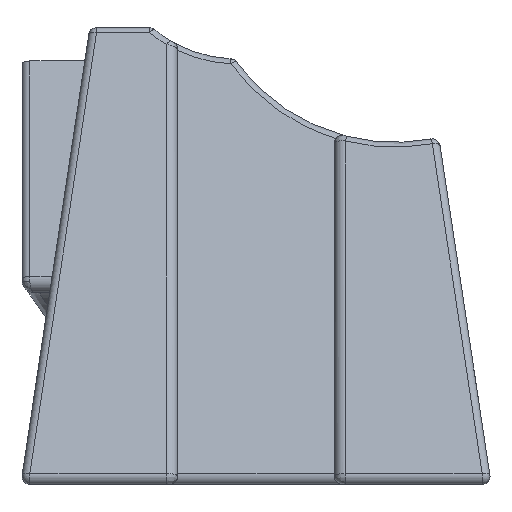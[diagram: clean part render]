
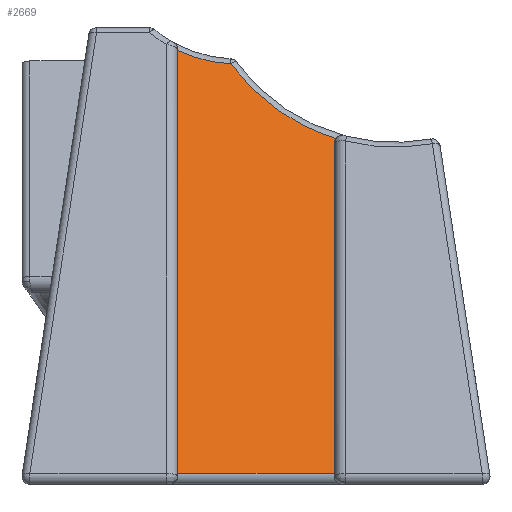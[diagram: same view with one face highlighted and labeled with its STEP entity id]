
A CAD part, top view. The second image highlights one B-rep face of the part: STEP entity #2669.
In plain terms, the highlighted planar face has unit normal (0, 0.375, 0.927).
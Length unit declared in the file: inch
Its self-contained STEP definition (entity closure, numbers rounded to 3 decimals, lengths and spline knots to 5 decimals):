
#122=ELLIPSE('',#2958,0.01079,0.01);
#123=ELLIPSE('',#2959,0.28042,0.26);
#124=ELLIPSE('',#2960,0.18975,0.17593);
#189=PLANE('',#2957);
#278=LINE('',#4767,#435);
#316=LINE('',#5097,#473);
#318=LINE('',#5103,#475);
#435=VECTOR('',#3390,0.3937);
#473=VECTOR('',#3580,0.3937);
#475=VECTOR('',#3586,0.3937);
#661=FACE_OUTER_BOUND('',#832,.T.);
#832=EDGE_LOOP('',(#2152,#2153,#2154,#2155,#2156,#2157));
#1212=VERTEX_POINT('',#4765);
#1213=VERTEX_POINT('',#4766);
#1272=VERTEX_POINT('',#5096);
#1274=VERTEX_POINT('',#5102);
#1275=VERTEX_POINT('',#5104);
#1276=VERTEX_POINT('',#5106);
#1500=EDGE_CURVE('',#1212,#1213,#278,.T.);
#1593=EDGE_CURVE('',#1213,#1272,#316,.T.);
#1596=EDGE_CURVE('',#1212,#1274,#318,.T.);
#1597=EDGE_CURVE('',#1275,#1274,#122,.T.);
#1598=EDGE_CURVE('',#1276,#1275,#123,.T.);
#1599=EDGE_CURVE('',#1272,#1276,#124,.T.);
#2152=ORIENTED_EDGE('',*,*,#1500,.F.);
#2153=ORIENTED_EDGE('',*,*,#1596,.T.);
#2154=ORIENTED_EDGE('',*,*,#1597,.F.);
#2155=ORIENTED_EDGE('',*,*,#1598,.F.);
#2156=ORIENTED_EDGE('',*,*,#1599,.F.);
#2157=ORIENTED_EDGE('',*,*,#1593,.F.);
#2669=ADVANCED_FACE('',(#661),#189,.F.);
#2957=AXIS2_PLACEMENT_3D('',#5101,#3584,#3585);
#2958=AXIS2_PLACEMENT_3D('',#5105,#3587,#3588);
#2959=AXIS2_PLACEMENT_3D('',#5107,#3589,#3590);
#2960=AXIS2_PLACEMENT_3D('',#5108,#3591,#3592);
#3390=DIRECTION('',(-1.,0.,0.));
#3580=DIRECTION('',(0.,0.927,-0.375));
#3584=DIRECTION('center_axis',(0.,-0.375,
-0.927));
#3585=DIRECTION('ref_axis',(-1.,0.,0.));
#3586=DIRECTION('',(0.,0.927,-0.375));
#3587=DIRECTION('center_axis',(0.,0.375,
0.927));
#3588=DIRECTION('ref_axis',(0.,0.927,-0.375));
#3589=DIRECTION('center_axis',(0.,0.375,
0.927));
#3590=DIRECTION('ref_axis',(0.,-0.927,0.375));
#3591=DIRECTION('center_axis',(0.,0.375,
0.927));
#3592=DIRECTION('ref_axis',(0.,-0.927,0.375));
#4765=CARTESIAN_POINT('',(-0.112,-0.23299,0.07796));
#4766=CARTESIAN_POINT('',(-0.312,-0.23299,0.07796));
#4767=CARTESIAN_POINT('',(-0.056,-0.23299,0.07796));
#5096=CARTESIAN_POINT('',(-0.312,0.30702,-0.14022));
#5097=CARTESIAN_POINT('',(-0.312,-0.26963,0.09276));
#5101=CARTESIAN_POINT('Origin',(-0.112,-0.26963,0.09276));
#5102=CARTESIAN_POINT('',(-0.112,0.18866,-0.0924));
#5103=CARTESIAN_POINT('',(-0.112,-0.26963,0.09276));
#5104=CARTESIAN_POINT('',(-0.10998,0.19469,-0.09484));
#5105=CARTESIAN_POINT('Origin',(-0.102,0.18866,-0.0924));
#5106=CARTESIAN_POINT('',(-0.24425,0.28992,-0.13331));
#5107=CARTESIAN_POINT('Origin',(-0.03445,0.44348,-0.19536));
#5108=CARTESIAN_POINT('Origin',(-0.23592,0.46565,-0.20431));
